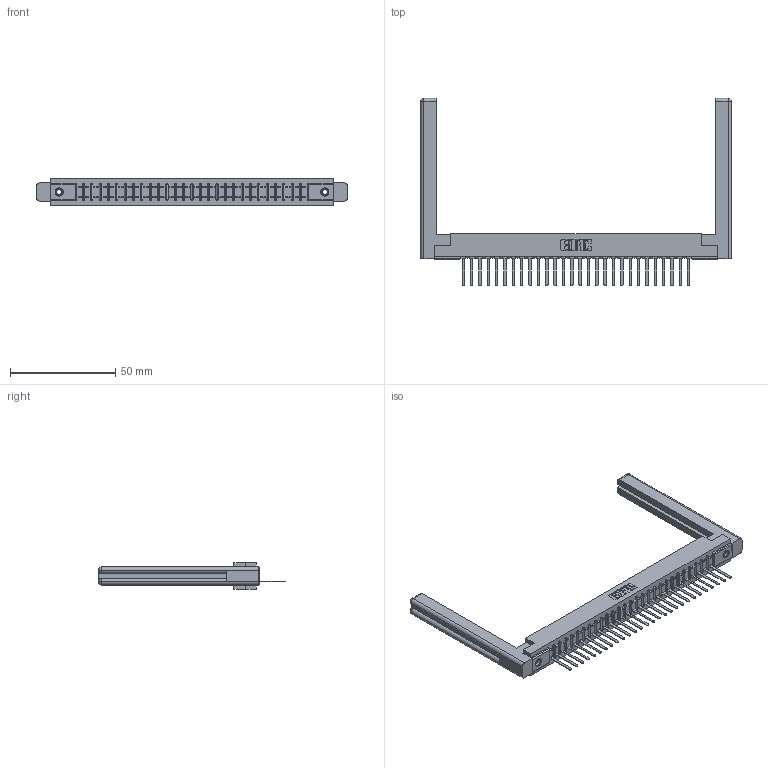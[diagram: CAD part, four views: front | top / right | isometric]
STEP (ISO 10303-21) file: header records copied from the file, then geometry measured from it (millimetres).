
FILE_DESCRIPTION (( 'STEP AP203' ), '1' );
FILE_NAME ('357-028-441-158.STEP', '2020-10-01T21:50:40', ( '' ), ( '' ), 'SwSTEP 2.0', 'SolidWorks 2020', '' );
FILE_SCHEMA (( 'CONFIG_CONTROL_DESIGN' ));
Length unit declared in the file: inch
Products named in the file (5): 307-290-002_541; 345-250-001_345-250-001-102; 307-220-058; 307 Part_.156 Dia Mounting Holes; 357-028-441-158
Assembly tree (33 placements, depth 2):
  357-028-441-158
    307 Part_.156 Dia Mounting Holes
    307-290-002_541  x28
    307-220-058  x2
    345-250-001_345-250-001-102  x2
Bounding box: 147.57 x 88.9 x 12.7 mm (x, y, z)
Volume: 22887.1 mm3; surface area: 24858.5 mm2
Topology: 33 solids, 33 shells, 2361 faces, 7173 edges, 4690 vertices
Faces by surface type: plane 1414, cylinder 865, sphere 58, torus 12, cone 12
Entity records: 29081 total; most frequent: CARTESIAN_POINT 4911, ORIENTED_EDGE 4840, DIRECTION 4738, EDGE_CURVE 2420, LINE 1844, VECTOR 1844, VERTEX_POINT 1566, AXIS2_PLACEMENT_3D 1447
